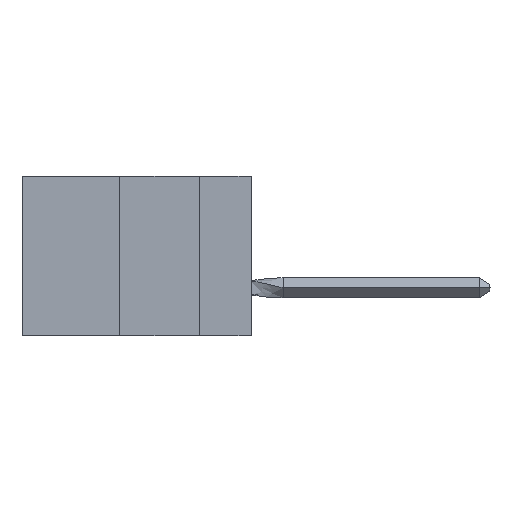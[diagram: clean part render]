
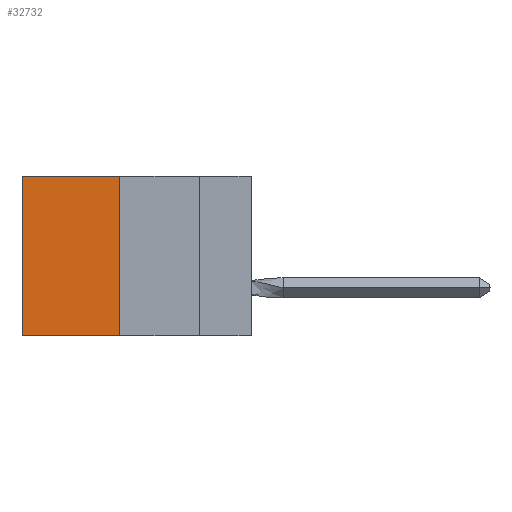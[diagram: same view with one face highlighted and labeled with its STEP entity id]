
A CAD part, left-side view. The second image highlights one B-rep face of the part: STEP entity #32732.
In plain terms, the highlighted planar face has unit normal (-1, 0, 0).
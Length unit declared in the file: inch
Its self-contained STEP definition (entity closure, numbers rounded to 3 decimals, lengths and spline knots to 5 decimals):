
#919 = VECTOR ( 'NONE', #34841, 39.37008 ) ;
#2262 = CARTESIAN_POINT ( 'NONE',  ( 0.305, 0.413, -0.5 ) ) ;
#2728 = DIRECTION ( 'NONE',  ( 0., 1., 0. ) ) ;
#3226 = CARTESIAN_POINT ( 'NONE',  ( 0.305, 0.72, -0.5 ) ) ;
#3685 = LINE ( 'NONE', #27664, #27162 ) ;
#4628 = CARTESIAN_POINT ( 'NONE',  ( 0.305, 0.72, -0.5 ) ) ;
#4802 = VERTEX_POINT ( 'NONE', #21958 ) ;
#5018 = CARTESIAN_POINT ( 'NONE',  ( 0.305, 0.72, 0. ) ) ;
#6327 = EDGE_CURVE ( 'NONE', #20846, #21142, #33008, .T. ) ;
#8272 = CARTESIAN_POINT ( 'NONE',  ( 0.305, 0.413, -0.5 ) ) ;
#8504 = CARTESIAN_POINT ( 'NONE',  ( 0.305, 0.413, 0. ) ) ;
#14239 = LINE ( 'NONE', #21403, #919 ) ;
#14625 = FACE_OUTER_BOUND ( 'NONE', #30483, .T. ) ;
#16015 = EDGE_CURVE ( 'NONE', #29825, #20846, #3685, .T. ) ;
#17689 = EDGE_CURVE ( 'NONE', #29825, #4802, #20689, .T. ) ;
#20689 = LINE ( 'NONE', #8272, #30019 ) ;
#20846 = VERTEX_POINT ( 'NONE', #5018 ) ;
#21142 = VERTEX_POINT ( 'NONE', #4628 ) ;
#21186 = PLANE ( 'NONE',  #22617 ) ;
#21403 = CARTESIAN_POINT ( 'NONE',  ( 0.305, 0.413, -0.5 ) ) ;
#21958 = CARTESIAN_POINT ( 'NONE',  ( 0.305, 0.413, -0.5 ) ) ;
#22617 = AXIS2_PLACEMENT_3D ( 'NONE', #2262, #31896, #29221 ) ;
#23289 = ORIENTED_EDGE ( 'NONE', *, *, #6327, .T. ) ;
#25076 = DIRECTION ( 'NONE',  ( 0., 0., -1. ) ) ;
#25177 = EDGE_CURVE ( 'NONE', #4802, #21142, #14239, .T. ) ;
#27162 = VECTOR ( 'NONE', #2728, 39.37008 ) ;
#27664 = CARTESIAN_POINT ( 'NONE',  ( 0.305, 0.413, 0. ) ) ;
#29221 = DIRECTION ( 'NONE',  ( 0., 0., -1. ) ) ;
#29760 = DIRECTION ( 'NONE',  ( 0., 0., -1. ) ) ;
#29825 = VERTEX_POINT ( 'NONE', #8504 ) ;
#30019 = VECTOR ( 'NONE', #29760, 39.37008 ) ;
#30483 = EDGE_LOOP ( 'NONE', ( #23289, #34516, #31089, #31959 ) ) ;
#31089 = ORIENTED_EDGE ( 'NONE', *, *, #17689, .F. ) ;
#31896 = DIRECTION ( 'NONE',  ( 1., 0., 0. ) ) ;
#31959 = ORIENTED_EDGE ( 'NONE', *, *, #16015, .T. ) ;
#32732 = ADVANCED_FACE ( 'NONE', ( #14625 ), #21186, .F. ) ;
#33008 = LINE ( 'NONE', #3226, #34693 ) ;
#34516 = ORIENTED_EDGE ( 'NONE', *, *, #25177, .F. ) ;
#34693 = VECTOR ( 'NONE', #25076, 39.37008 ) ;
#34841 = DIRECTION ( 'NONE',  ( 0., 1., 0. ) ) ;
